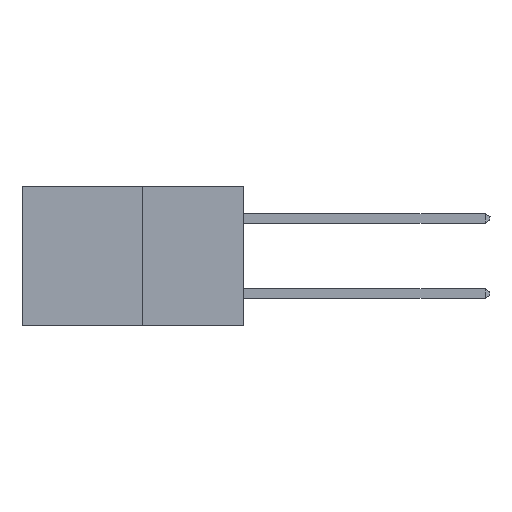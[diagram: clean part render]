
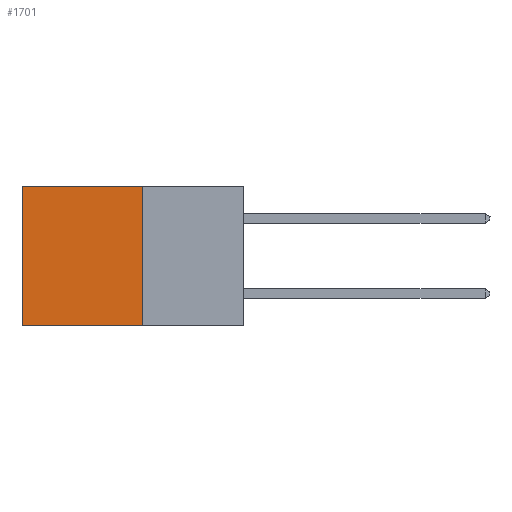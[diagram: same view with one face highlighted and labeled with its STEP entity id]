
A CAD part, left-side view. The second image highlights one B-rep face of the part: STEP entity #1701.
In plain terms, the highlighted planar face has unit normal (-1, 0, 0).
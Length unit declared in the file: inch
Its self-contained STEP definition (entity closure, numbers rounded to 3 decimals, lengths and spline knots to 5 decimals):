
#221 = LINE ( 'NONE', #4681, #8265 ) ;
#357 = CARTESIAN_POINT ( 'NONE',  ( 0.277, 0.27, 0. ) ) ;
#555 = CARTESIAN_POINT ( 'NONE',  ( 0.277, 0.27, -0.37 ) ) ;
#686 = EDGE_CURVE ( 'NONE', #3384, #2070, #9936, .T. ) ;
#726 = DIRECTION ( 'NONE',  ( 0., 0., -1. ) ) ;
#894 = DIRECTION ( 'NONE',  ( 0., 0., -1. ) ) ;
#1054 = CARTESIAN_POINT ( 'NONE',  ( 0.277, 0.59, -0.37 ) ) ;
#1701 = ADVANCED_FACE ( 'NONE', ( #4250 ), #8050, .F. ) ;
#2070 = VERTEX_POINT ( 'NONE', #3386 ) ;
#2312 = DIRECTION ( 'NONE',  ( 0., 0., -1. ) ) ;
#2460 = VERTEX_POINT ( 'NONE', #6537 ) ;
#2778 = EDGE_CURVE ( 'NONE', #2070, #5147, #221, .T. ) ;
#2962 = DIRECTION ( 'NONE',  ( 1., 0., 0. ) ) ;
#3038 = LINE ( 'NONE', #3988, #7118 ) ;
#3384 = VERTEX_POINT ( 'NONE', #8025 ) ;
#3386 = CARTESIAN_POINT ( 'NONE',  ( 0.277, 0.59, 0. ) ) ;
#3762 = AXIS2_PLACEMENT_3D ( 'NONE', #555, #2962, #2312 ) ;
#3988 = CARTESIAN_POINT ( 'NONE',  ( 0.277, 0.27, -0.37 ) ) ;
#4168 = DIRECTION ( 'NONE',  ( 0., 1., 0. ) ) ;
#4196 = ORIENTED_EDGE ( 'NONE', *, *, #686, .T. ) ;
#4219 = EDGE_LOOP ( 'NONE', ( #8638, #7164, #4767, #4196 ) ) ;
#4250 = FACE_OUTER_BOUND ( 'NONE', #4219, .T. ) ;
#4648 = VECTOR ( 'NONE', #894, 39.37008 ) ;
#4681 = CARTESIAN_POINT ( 'NONE',  ( 0.277, 0.59, -0.37 ) ) ;
#4767 = ORIENTED_EDGE ( 'NONE', *, *, #9343, .F. ) ;
#5147 = VERTEX_POINT ( 'NONE', #1054 ) ;
#5970 = DIRECTION ( 'NONE',  ( 0., 1., 0. ) ) ;
#6205 = CARTESIAN_POINT ( 'NONE',  ( 0.277, 0.27, -0.37 ) ) ;
#6537 = CARTESIAN_POINT ( 'NONE',  ( 0.277, 0.27, -0.37 ) ) ;
#7118 = VECTOR ( 'NONE', #4168, 39.37008 ) ;
#7164 = ORIENTED_EDGE ( 'NONE', *, *, #8883, .F. ) ;
#8025 = CARTESIAN_POINT ( 'NONE',  ( 0.277, 0.27, 0. ) ) ;
#8050 = PLANE ( 'NONE',  #3762 ) ;
#8265 = VECTOR ( 'NONE', #726, 39.37008 ) ;
#8568 = LINE ( 'NONE', #6205, #4648 ) ;
#8638 = ORIENTED_EDGE ( 'NONE', *, *, #2778, .T. ) ;
#8883 = EDGE_CURVE ( 'NONE', #2460, #5147, #3038, .T. ) ;
#9343 = EDGE_CURVE ( 'NONE', #3384, #2460, #8568, .T. ) ;
#9493 = VECTOR ( 'NONE', #5970, 39.37008 ) ;
#9936 = LINE ( 'NONE', #357, #9493 ) ;
